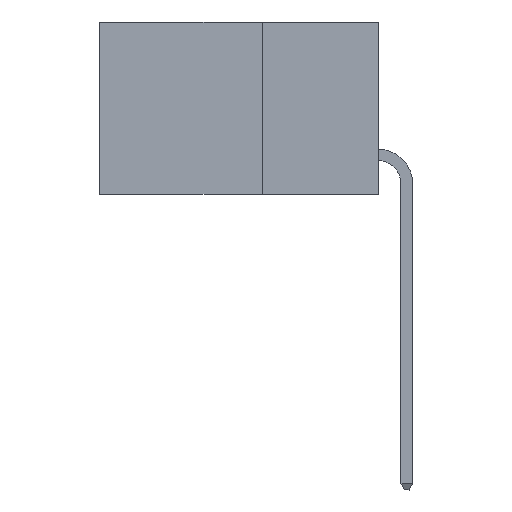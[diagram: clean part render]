
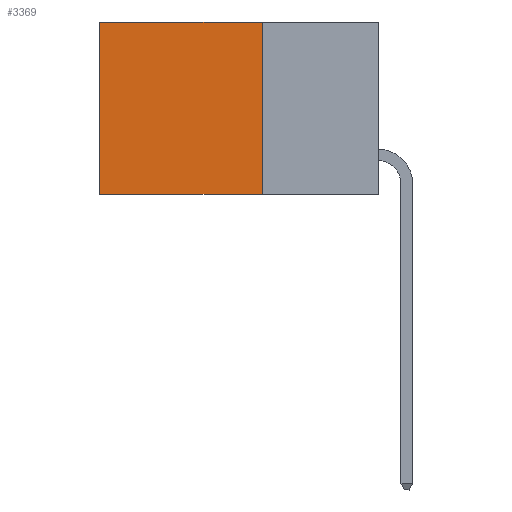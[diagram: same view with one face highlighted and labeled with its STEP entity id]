
A CAD part, left-side view. The second image highlights one B-rep face of the part: STEP entity #3369.
In plain terms, the highlighted planar face has unit normal (-1, 0, 0).
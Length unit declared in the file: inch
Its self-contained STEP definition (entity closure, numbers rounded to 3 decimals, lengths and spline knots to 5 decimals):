
#284 = CARTESIAN_POINT ( 'NONE',  ( 0.2615, 0.6, 0. ) ) ;
#608 = EDGE_LOOP ( 'NONE', ( #699, #4819, #4360, #2866 ) ) ;
#621 = VECTOR ( 'NONE', #1530, 39.37008 ) ;
#699 = ORIENTED_EDGE ( 'NONE', *, *, #2370, .T. ) ;
#751 = EDGE_CURVE ( 'NONE', #4007, #5849, #6119, .T. ) ;
#1530 = DIRECTION ( 'NONE',  ( 0., 1., 0. ) ) ;
#1542 = CARTESIAN_POINT ( 'NONE',  ( 0.2615, 0.25, -0.37 ) ) ;
#1663 = AXIS2_PLACEMENT_3D ( 'NONE', #3157, #9386, #6257 ) ;
#1809 = CARTESIAN_POINT ( 'NONE',  ( 0.2615, 0.6, -0.37 ) ) ;
#2001 = VECTOR ( 'NONE', #2262, 39.37008 ) ;
#2258 = CARTESIAN_POINT ( 'NONE',  ( 0.2615, 0.25, -0.37 ) ) ;
#2262 = DIRECTION ( 'NONE',  ( 0., 0., -1. ) ) ;
#2370 = EDGE_CURVE ( 'NONE', #6253, #3513, #8809, .T. ) ;
#2688 = CARTESIAN_POINT ( 'NONE',  ( 0.2615, 0.6, -0.37 ) ) ;
#2866 = ORIENTED_EDGE ( 'NONE', *, *, #7753, .T. ) ;
#3116 = LINE ( 'NONE', #2258, #6702 ) ;
#3157 = CARTESIAN_POINT ( 'NONE',  ( 0.2615, 0.25, -0.37 ) ) ;
#3345 = PLANE ( 'NONE',  #1663 ) ;
#3369 = ADVANCED_FACE ( 'NONE', ( #5642 ), #3345, .F. ) ;
#3513 = VERTEX_POINT ( 'NONE', #2688 ) ;
#3831 = LINE ( 'NONE', #8693, #621 ) ;
#4007 = VERTEX_POINT ( 'NONE', #5680 ) ;
#4360 = ORIENTED_EDGE ( 'NONE', *, *, #751, .F. ) ;
#4729 = EDGE_CURVE ( 'NONE', #5849, #3513, #3116, .T. ) ;
#4819 = ORIENTED_EDGE ( 'NONE', *, *, #4729, .F. ) ;
#5642 = FACE_OUTER_BOUND ( 'NONE', #608, .T. ) ;
#5680 = CARTESIAN_POINT ( 'NONE',  ( 0.2615, 0.25, 0. ) ) ;
#5849 = VERTEX_POINT ( 'NONE', #7709 ) ;
#6119 = LINE ( 'NONE', #1542, #2001 ) ;
#6253 = VERTEX_POINT ( 'NONE', #284 ) ;
#6257 = DIRECTION ( 'NONE',  ( 0., 0., -1. ) ) ;
#6480 = DIRECTION ( 'NONE',  ( 0., 0., -1. ) ) ;
#6702 = VECTOR ( 'NONE', #7868, 39.37008 ) ;
#7709 = CARTESIAN_POINT ( 'NONE',  ( 0.2615, 0.25, -0.37 ) ) ;
#7753 = EDGE_CURVE ( 'NONE', #4007, #6253, #3831, .T. ) ;
#7868 = DIRECTION ( 'NONE',  ( 0., 1., 0. ) ) ;
#8693 = CARTESIAN_POINT ( 'NONE',  ( 0.2615, 0.25, 0. ) ) ;
#8809 = LINE ( 'NONE', #1809, #8920 ) ;
#8920 = VECTOR ( 'NONE', #6480, 39.37008 ) ;
#9386 = DIRECTION ( 'NONE',  ( 1., 0., 0. ) ) ;
